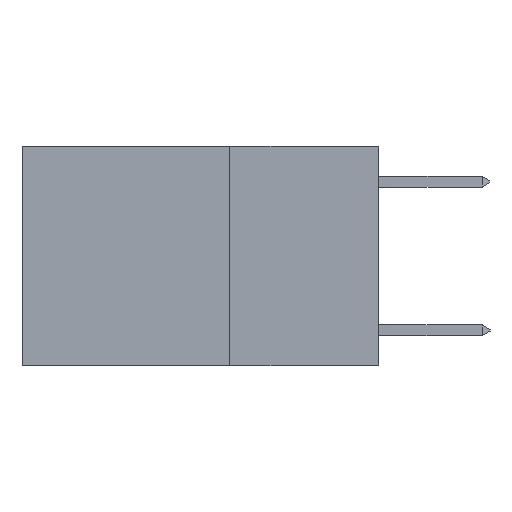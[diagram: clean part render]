
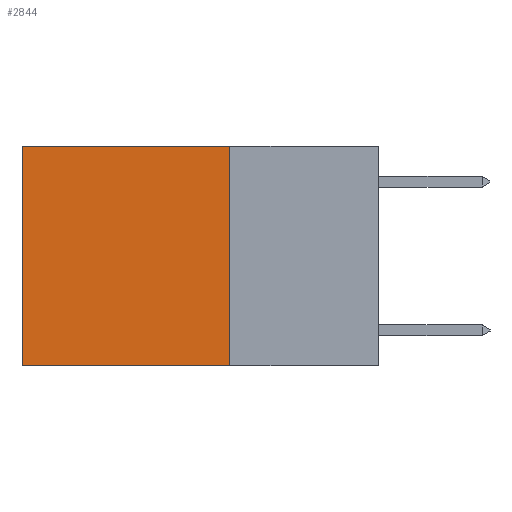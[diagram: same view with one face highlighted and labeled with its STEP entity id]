
A CAD part, left-side view. The second image highlights one B-rep face of the part: STEP entity #2844.
In plain terms, the highlighted planar face has unit normal (-1, 0, 0).
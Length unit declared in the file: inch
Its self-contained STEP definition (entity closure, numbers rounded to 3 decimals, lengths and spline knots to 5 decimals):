
#241 = ORIENTED_EDGE ( 'NONE', *, *, #8462, .T. ) ;
#574 = VECTOR ( 'NONE', #4604, 39.37008 ) ;
#1013 = LINE ( 'NONE', #4803, #7919 ) ;
#1110 = VERTEX_POINT ( 'NONE', #5994 ) ;
#1305 = CARTESIAN_POINT ( 'NONE',  ( 0.2625, 0.25, -0.37 ) ) ;
#1549 = VECTOR ( 'NONE', #5814, 39.37008 ) ;
#1649 = EDGE_CURVE ( 'NONE', #2537, #8660, #3361, .T. ) ;
#1786 = CARTESIAN_POINT ( 'NONE',  ( 0.2625, 0.25, -0.37 ) ) ;
#2032 = ORIENTED_EDGE ( 'NONE', *, *, #5473, .T. ) ;
#2236 = LINE ( 'NONE', #8531, #574 ) ;
#2537 = VERTEX_POINT ( 'NONE', #1305 ) ;
#2805 = LINE ( 'NONE', #4280, #4190 ) ;
#2808 = CARTESIAN_POINT ( 'NONE',  ( 0.2625, 0.6, 0. ) ) ;
#2844 = ADVANCED_FACE ( 'NONE', ( #5205 ), #6281, .F. ) ;
#2969 = DIRECTION ( 'NONE',  ( 1., 0., 0. ) ) ;
#3361 = LINE ( 'NONE', #1786, #1549 ) ;
#3495 = DIRECTION ( 'NONE',  ( 0., 1., 0. ) ) ;
#3718 = EDGE_CURVE ( 'NONE', #1110, #2537, #2236, .T. ) ;
#3930 = VERTEX_POINT ( 'NONE', #2808 ) ;
#4190 = VECTOR ( 'NONE', #8201, 39.37008 ) ;
#4280 = CARTESIAN_POINT ( 'NONE',  ( 0.2625, 0.6, 0. ) ) ;
#4604 = DIRECTION ( 'NONE',  ( 0., 0., -1. ) ) ;
#4803 = CARTESIAN_POINT ( 'NONE',  ( 0.2625, 0.25, 0. ) ) ;
#4903 = ORIENTED_EDGE ( 'NONE', *, *, #3718, .F. ) ;
#5205 = FACE_OUTER_BOUND ( 'NONE', #6382, .T. ) ;
#5473 = EDGE_CURVE ( 'NONE', #1110, #3930, #1013, .T. ) ;
#5550 = AXIS2_PLACEMENT_3D ( 'NONE', #5626, #2969, #7605 ) ;
#5626 = CARTESIAN_POINT ( 'NONE',  ( 0.2625, 0.25, 0. ) ) ;
#5814 = DIRECTION ( 'NONE',  ( 0., 1., 0. ) ) ;
#5994 = CARTESIAN_POINT ( 'NONE',  ( 0.2625, 0.25, 0. ) ) ;
#6281 = PLANE ( 'NONE',  #5550 ) ;
#6346 = CARTESIAN_POINT ( 'NONE',  ( 0.2625, 0.6, -0.37 ) ) ;
#6382 = EDGE_LOOP ( 'NONE', ( #241, #8085, #4903, #2032 ) ) ;
#7605 = DIRECTION ( 'NONE',  ( 0., 0., -1. ) ) ;
#7919 = VECTOR ( 'NONE', #3495, 39.37008 ) ;
#8085 = ORIENTED_EDGE ( 'NONE', *, *, #1649, .F. ) ;
#8201 = DIRECTION ( 'NONE',  ( 0., 0., -1. ) ) ;
#8462 = EDGE_CURVE ( 'NONE', #3930, #8660, #2805, .T. ) ;
#8531 = CARTESIAN_POINT ( 'NONE',  ( 0.2625, 0.25, 0. ) ) ;
#8660 = VERTEX_POINT ( 'NONE', #6346 ) ;
